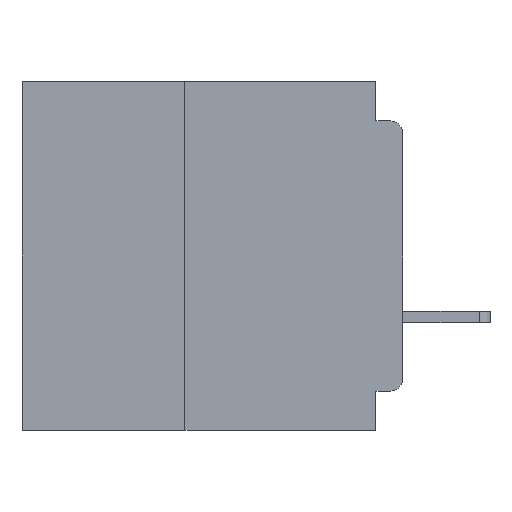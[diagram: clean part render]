
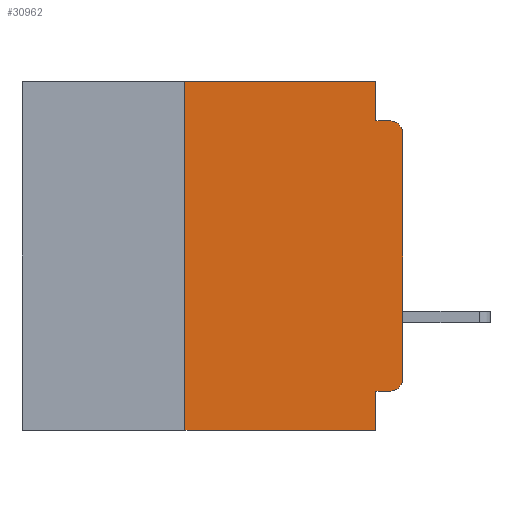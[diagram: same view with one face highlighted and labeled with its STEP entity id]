
A CAD part, left-side view. The second image highlights one B-rep face of the part: STEP entity #30962.
In plain terms, the highlighted planar face has unit normal (-1, 0, 0).
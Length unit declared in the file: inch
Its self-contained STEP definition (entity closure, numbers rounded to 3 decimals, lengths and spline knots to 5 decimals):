
#981 = CARTESIAN_POINT ( 'NONE',  ( 0., 0.015, -0.355 ) ) ;
#1173 = VECTOR ( 'NONE', #33244, 39.37008 ) ;
#2982 = CARTESIAN_POINT ( 'NONE',  ( 0., 0.437, 0. ) ) ;
#3058 = VERTEX_POINT ( 'NONE', #21235 ) ;
#3247 = VERTEX_POINT ( 'NONE', #15141 ) ;
#3839 = CIRCLE ( 'NONE', #37630, 0.015 ) ;
#4950 = ORIENTED_EDGE ( 'NONE', *, *, #26379, .F. ) ;
#5353 = LINE ( 'NONE', #59397, #43977 ) ;
#5913 = VECTOR ( 'NONE', #44154, 39.37008 ) ;
#6487 = CARTESIAN_POINT ( 'NONE',  ( 0., 0.031, -0.4 ) ) ;
#7369 = ORIENTED_EDGE ( 'NONE', *, *, #53630, .F. ) ;
#8368 = CARTESIAN_POINT ( 'NONE',  ( 0., 0.437, -0.4 ) ) ;
#8427 = VERTEX_POINT ( 'NONE', #25661 ) ;
#8931 = CARTESIAN_POINT ( 'NONE',  ( 0., 0., -0.355 ) ) ;
#8966 = VECTOR ( 'NONE', #63465, 39.37008 ) ;
#9379 = CARTESIAN_POINT ( 'NONE',  ( 0., 0.015, -0.34 ) ) ;
#9896 = DIRECTION ( 'NONE',  ( 0., 0., 1. ) ) ;
#11118 = CARTESIAN_POINT ( 'NONE',  ( 0., 0.25, 0. ) ) ;
#12061 = ORIENTED_EDGE ( 'NONE', *, *, #25820, .T. ) ;
#13634 = ORIENTED_EDGE ( 'NONE', *, *, #38824, .T. ) ;
#14313 = CIRCLE ( 'NONE', #54149, 0.015 ) ;
#14434 = DIRECTION ( 'NONE',  ( 0., 0., -1. ) ) ;
#14619 = LINE ( 'NONE', #2982, #1173 ) ;
#15004 = LINE ( 'NONE', #40044, #43366 ) ;
#15141 = CARTESIAN_POINT ( 'NONE',  ( 0., 0.031, -0.355 ) ) ;
#15236 = ORIENTED_EDGE ( 'NONE', *, *, #52472, .F. ) ;
#15741 = VECTOR ( 'NONE', #57306, 39.37008 ) ;
#18205 = DIRECTION ( 'NONE',  ( -1., 0., 0. ) ) ;
#19933 = CARTESIAN_POINT ( 'NONE',  ( 0., 0.437, 0. ) ) ;
#21235 = CARTESIAN_POINT ( 'NONE',  ( 0., 0., -0.34 ) ) ;
#21589 = ORIENTED_EDGE ( 'NONE', *, *, #22556, .T. ) ;
#21708 = DIRECTION ( 'NONE',  ( 0., 0., -1. ) ) ;
#21933 = EDGE_CURVE ( 'NONE', #3058, #64506, #15004, .T. ) ;
#22190 = CARTESIAN_POINT ( 'NONE',  ( 0., 0.25, -0.4 ) ) ;
#22556 = EDGE_CURVE ( 'NONE', #64625, #3058, #3839, .T. ) ;
#24359 = DIRECTION ( 'NONE',  ( 0., 0., -1. ) ) ;
#25661 = CARTESIAN_POINT ( 'NONE',  ( 0., 0.25, -0.4 ) ) ;
#25820 = EDGE_CURVE ( 'NONE', #64506, #53607, #14313, .T. ) ;
#26379 = EDGE_CURVE ( 'NONE', #54499, #53607, #30935, .T. ) ;
#27460 = VECTOR ( 'NONE', #21708, 39.37008 ) ;
#27657 = EDGE_CURVE ( 'NONE', #8427, #58757, #42530, .T. ) ;
#28533 = CARTESIAN_POINT ( 'NONE',  ( 0., 0., -0.045 ) ) ;
#29648 = EDGE_CURVE ( 'NONE', #64625, #3247, #60954, .T. ) ;
#30098 = DIRECTION ( 'NONE',  ( 1., 0., 0. ) ) ;
#30935 = LINE ( 'NONE', #28533, #56041 ) ;
#30962 = ADVANCED_FACE ( 'NONE', ( #56094 ), #59886, .F. ) ;
#33244 = DIRECTION ( 'NONE',  ( 0., -1., 0. ) ) ;
#33610 = DIRECTION ( 'NONE',  ( 0., -1., 0. ) ) ;
#34235 = EDGE_CURVE ( 'NONE', #53459, #54499, #54180, .T. ) ;
#37340 = LINE ( 'NONE', #8368, #8966 ) ;
#37630 = AXIS2_PLACEMENT_3D ( 'NONE', #9379, #44585, #14434 ) ;
#38824 = EDGE_CURVE ( 'NONE', #8427, #43109, #37340, .T. ) ;
#38900 = ORIENTED_EDGE ( 'NONE', *, *, #27657, .F. ) ;
#40044 = CARTESIAN_POINT ( 'NONE',  ( 0., 0., 0. ) ) ;
#42037 = ORIENTED_EDGE ( 'NONE', *, *, #29648, .F. ) ;
#42043 = CARTESIAN_POINT ( 'NONE',  ( 0., 0.031, 0. ) ) ;
#42530 = LINE ( 'NONE', #22190, #15741 ) ;
#43109 = VERTEX_POINT ( 'NONE', #6487 ) ;
#43366 = VECTOR ( 'NONE', #9896, 39.37008 ) ;
#43977 = VECTOR ( 'NONE', #24359, 39.37008 ) ;
#44154 = DIRECTION ( 'NONE',  ( 0., 1., 0. ) ) ;
#44585 = DIRECTION ( 'NONE',  ( -1., 0., 0. ) ) ;
#45861 = CARTESIAN_POINT ( 'NONE',  ( 0., 0.031, -0.045 ) ) ;
#48363 = CARTESIAN_POINT ( 'NONE',  ( 0., 0.015, -0.06 ) ) ;
#49058 = ORIENTED_EDGE ( 'NONE', *, *, #21933, .T. ) ;
#52472 = EDGE_CURVE ( 'NONE', #3247, #43109, #5353, .T. ) ;
#53392 = DIRECTION ( 'NONE',  ( 0., 0., -1. ) ) ;
#53459 = VERTEX_POINT ( 'NONE', #42043 ) ;
#53607 = VERTEX_POINT ( 'NONE', #57982 ) ;
#53630 = EDGE_CURVE ( 'NONE', #58757, #53459, #14619, .T. ) ;
#54149 = AXIS2_PLACEMENT_3D ( 'NONE', #48363, #18205, #53392 ) ;
#54180 = LINE ( 'NONE', #56824, #27460 ) ;
#54499 = VERTEX_POINT ( 'NONE', #45861 ) ;
#55382 = CARTESIAN_POINT ( 'NONE',  ( 0., 0., -0.06 ) ) ;
#56041 = VECTOR ( 'NONE', #33610, 39.37008 ) ;
#56094 = FACE_OUTER_BOUND ( 'NONE', #58434, .T. ) ;
#56824 = CARTESIAN_POINT ( 'NONE',  ( 0., 0.031, 0. ) ) ;
#57306 = DIRECTION ( 'NONE',  ( 0., 0., 1. ) ) ;
#57982 = CARTESIAN_POINT ( 'NONE',  ( 0., 0.015, -0.045 ) ) ;
#58434 = EDGE_LOOP ( 'NONE', ( #49058, #12061, #4950, #64670, #7369, #38900, #13634, #15236, #42037, #21589 ) ) ;
#58757 = VERTEX_POINT ( 'NONE', #11118 ) ;
#59358 = AXIS2_PLACEMENT_3D ( 'NONE', #19933, #30098, #65081 ) ;
#59397 = CARTESIAN_POINT ( 'NONE',  ( 0., 0.031, -0.4 ) ) ;
#59886 = PLANE ( 'NONE',  #59358 ) ;
#60954 = LINE ( 'NONE', #8931, #5913 ) ;
#63465 = DIRECTION ( 'NONE',  ( 0., -1., 0. ) ) ;
#64506 = VERTEX_POINT ( 'NONE', #55382 ) ;
#64625 = VERTEX_POINT ( 'NONE', #981 ) ;
#64670 = ORIENTED_EDGE ( 'NONE', *, *, #34235, .F. ) ;
#65081 = DIRECTION ( 'NONE',  ( 0., 0., -1. ) ) ;
